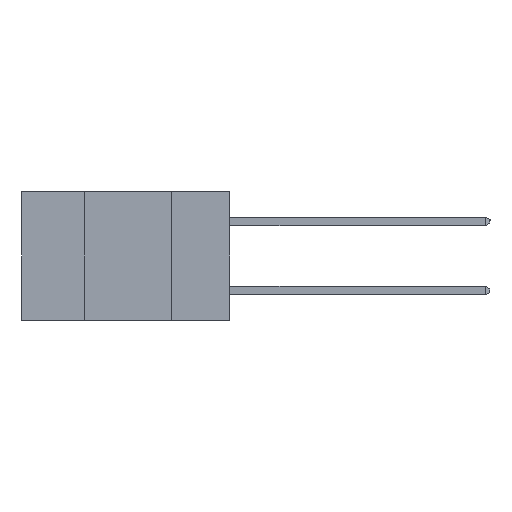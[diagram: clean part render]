
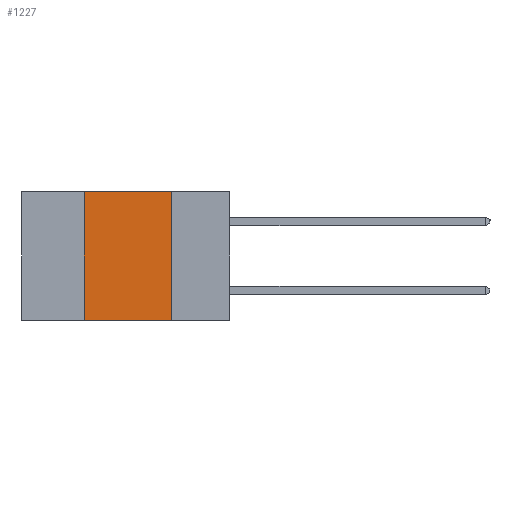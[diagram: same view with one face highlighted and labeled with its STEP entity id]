
A CAD part, left-side view. The second image highlights one B-rep face of the part: STEP entity #1227.
In plain terms, the highlighted planar face has unit normal (-1, 0, 0).
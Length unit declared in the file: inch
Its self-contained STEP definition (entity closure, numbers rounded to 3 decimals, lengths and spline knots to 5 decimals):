
#223 = VECTOR ( 'NONE', #4043, 39.37008 ) ;
#286 = EDGE_CURVE ( 'NONE', #3743, #5013, #13268, .T. ) ;
#828 = CARTESIAN_POINT ( 'NONE',  ( 0., 0.42, 0. ) ) ;
#1114 = CARTESIAN_POINT ( 'NONE',  ( 0., 0.42, -0.37 ) ) ;
#1227 = ADVANCED_FACE ( 'NONE', ( #7977 ), #11053, .F. ) ;
#1452 = CARTESIAN_POINT ( 'NONE',  ( 0., 0.6, 0. ) ) ;
#1604 = LINE ( 'NONE', #6431, #223 ) ;
#1692 = LINE ( 'NONE', #2864, #7181 ) ;
#2199 = ORIENTED_EDGE ( 'NONE', *, *, #5810, .F. ) ;
#2864 = CARTESIAN_POINT ( 'NONE',  ( 0., 0.17, -0.37 ) ) ;
#2995 = LINE ( 'NONE', #10379, #15551 ) ;
#3743 = VERTEX_POINT ( 'NONE', #3965 ) ;
#3751 = DIRECTION ( 'NONE',  ( 0., 0., -1. ) ) ;
#3795 = EDGE_CURVE ( 'NONE', #5013, #5780, #1604, .T. ) ;
#3965 = CARTESIAN_POINT ( 'NONE',  ( 0., 0.42, -0.37 ) ) ;
#4043 = DIRECTION ( 'NONE',  ( 0., -1., 0. ) ) ;
#5013 = VERTEX_POINT ( 'NONE', #828 ) ;
#5780 = VERTEX_POINT ( 'NONE', #12563 ) ;
#5810 = EDGE_CURVE ( 'NONE', #5780, #9925, #1692, .T. ) ;
#5967 = DIRECTION ( 'NONE',  ( 0., 0., 1. ) ) ;
#6431 = CARTESIAN_POINT ( 'NONE',  ( 0., 0.6, 0. ) ) ;
#6917 = DIRECTION ( 'NONE',  ( 0., 0., -1. ) ) ;
#7181 = VECTOR ( 'NONE', #6917, 39.37008 ) ;
#7192 = EDGE_CURVE ( 'NONE', #3743, #9925, #2995, .T. ) ;
#7699 = ORIENTED_EDGE ( 'NONE', *, *, #7192, .T. ) ;
#7817 = DIRECTION ( 'NONE',  ( 0., -1., 0. ) ) ;
#7977 = FACE_OUTER_BOUND ( 'NONE', #8105, .T. ) ;
#8105 = EDGE_LOOP ( 'NONE', ( #2199, #8616, #13396, #7699 ) ) ;
#8616 = ORIENTED_EDGE ( 'NONE', *, *, #3795, .F. ) ;
#9925 = VERTEX_POINT ( 'NONE', #14191 ) ;
#10379 = CARTESIAN_POINT ( 'NONE',  ( 0., 0.6, -0.37 ) ) ;
#11053 = PLANE ( 'NONE',  #15189 ) ;
#11925 = VECTOR ( 'NONE', #5967, 39.37008 ) ;
#12563 = CARTESIAN_POINT ( 'NONE',  ( 0., 0.17, 0. ) ) ;
#13268 = LINE ( 'NONE', #1114, #11925 ) ;
#13396 = ORIENTED_EDGE ( 'NONE', *, *, #286, .F. ) ;
#14191 = CARTESIAN_POINT ( 'NONE',  ( 0., 0.17, -0.37 ) ) ;
#14616 = DIRECTION ( 'NONE',  ( 1., 0., 0. ) ) ;
#15189 = AXIS2_PLACEMENT_3D ( 'NONE', #1452, #14616, #3751 ) ;
#15551 = VECTOR ( 'NONE', #7817, 39.37008 ) ;
